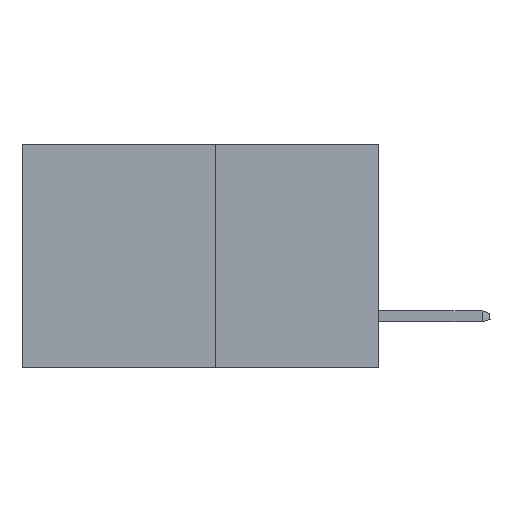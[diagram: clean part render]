
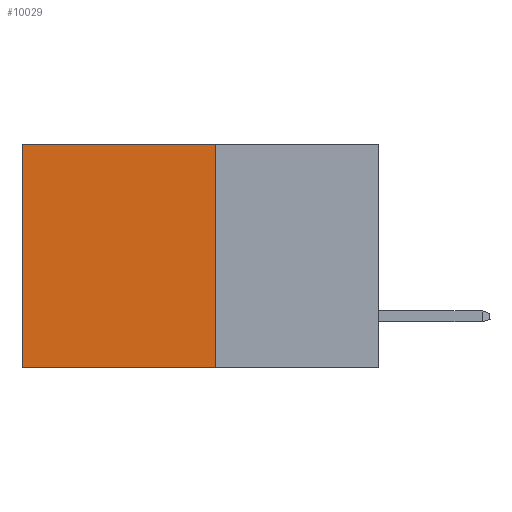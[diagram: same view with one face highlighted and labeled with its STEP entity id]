
A CAD part, left-side view. The second image highlights one B-rep face of the part: STEP entity #10029.
In plain terms, the highlighted planar face has unit normal (-1, 0, 0).
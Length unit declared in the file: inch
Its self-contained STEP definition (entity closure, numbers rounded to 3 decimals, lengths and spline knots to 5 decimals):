
#538 = EDGE_CURVE ( 'NONE', #3381, #7280, #10383, .T. ) ;
#1501 = CARTESIAN_POINT ( 'NONE',  ( 0.277, 0.27, -0.37 ) ) ;
#1766 = CARTESIAN_POINT ( 'NONE',  ( 0.277, 0.27, -0.37 ) ) ;
#2104 = PLANE ( 'NONE',  #5399 ) ;
#2286 = DIRECTION ( 'NONE',  ( 0., 1., 0. ) ) ;
#2487 = ORIENTED_EDGE ( 'NONE', *, *, #11829, .F. ) ;
#3381 = VERTEX_POINT ( 'NONE', #8995 ) ;
#3537 = DIRECTION ( 'NONE',  ( 0., 1., 0. ) ) ;
#3626 = CARTESIAN_POINT ( 'NONE',  ( 0.277, 0.27, 0. ) ) ;
#4002 = LINE ( 'NONE', #1501, #10790 ) ;
#4118 = VERTEX_POINT ( 'NONE', #11572 ) ;
#4135 = CARTESIAN_POINT ( 'NONE',  ( 0.277, 0.27, -0.37 ) ) ;
#4181 = DIRECTION ( 'NONE',  ( 0., 0., -1. ) ) ;
#4796 = VECTOR ( 'NONE', #11953, 39.37008 ) ;
#4893 = CARTESIAN_POINT ( 'NONE',  ( 0.277, 0.59, -0.37 ) ) ;
#5021 = DIRECTION ( 'NONE',  ( 0., 0., -1. ) ) ;
#5399 = AXIS2_PLACEMENT_3D ( 'NONE', #4135, #10217, #4181 ) ;
#6173 = EDGE_CURVE ( 'NONE', #9866, #4118, #4002, .T. ) ;
#7111 = EDGE_LOOP ( 'NONE', ( #13226, #9415, #2487, #7439 ) ) ;
#7280 = VERTEX_POINT ( 'NONE', #10377 ) ;
#7439 = ORIENTED_EDGE ( 'NONE', *, *, #538, .T. ) ;
#8906 = LINE ( 'NONE', #12084, #9206 ) ;
#8995 = CARTESIAN_POINT ( 'NONE',  ( 0.277, 0.27, 0. ) ) ;
#9206 = VECTOR ( 'NONE', #5021, 39.37008 ) ;
#9415 = ORIENTED_EDGE ( 'NONE', *, *, #6173, .F. ) ;
#9420 = FACE_OUTER_BOUND ( 'NONE', #7111, .T. ) ;
#9866 = VERTEX_POINT ( 'NONE', #1766 ) ;
#10029 = ADVANCED_FACE ( 'NONE', ( #9420 ), #2104, .F. ) ;
#10217 = DIRECTION ( 'NONE',  ( 1., 0., 0. ) ) ;
#10377 = CARTESIAN_POINT ( 'NONE',  ( 0.277, 0.59, 0. ) ) ;
#10383 = LINE ( 'NONE', #3626, #12757 ) ;
#10790 = VECTOR ( 'NONE', #2286, 39.37008 ) ;
#11572 = CARTESIAN_POINT ( 'NONE',  ( 0.277, 0.59, -0.37 ) ) ;
#11743 = EDGE_CURVE ( 'NONE', #7280, #4118, #12213, .T. ) ;
#11829 = EDGE_CURVE ( 'NONE', #3381, #9866, #8906, .T. ) ;
#11953 = DIRECTION ( 'NONE',  ( 0., 0., -1. ) ) ;
#12084 = CARTESIAN_POINT ( 'NONE',  ( 0.277, 0.27, -0.37 ) ) ;
#12213 = LINE ( 'NONE', #4893, #4796 ) ;
#12757 = VECTOR ( 'NONE', #3537, 39.37008 ) ;
#13226 = ORIENTED_EDGE ( 'NONE', *, *, #11743, .T. ) ;
